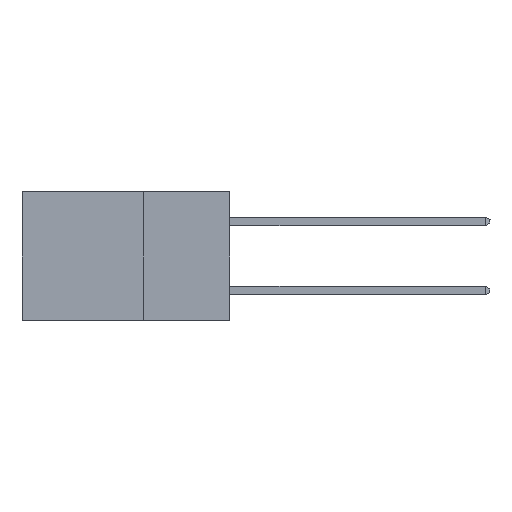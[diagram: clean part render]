
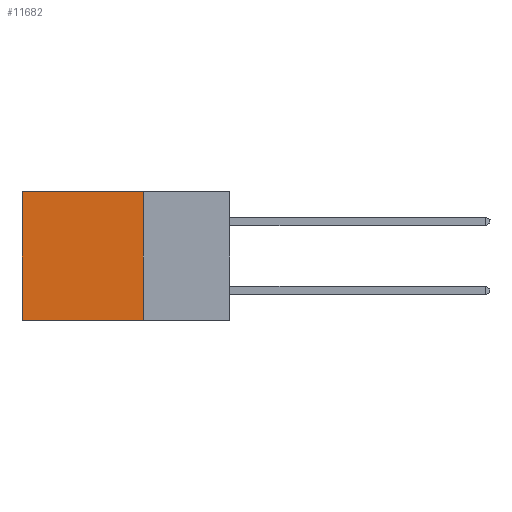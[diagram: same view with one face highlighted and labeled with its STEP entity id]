
A CAD part, left-side view. The second image highlights one B-rep face of the part: STEP entity #11682.
In plain terms, the highlighted planar face has unit normal (-1, 0, 0).
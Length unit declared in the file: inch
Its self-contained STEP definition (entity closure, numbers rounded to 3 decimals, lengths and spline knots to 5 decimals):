
#740 = VERTEX_POINT ( 'NONE', #20761 ) ;
#2469 = VECTOR ( 'NONE', #8230, 39.37008 ) ;
#3458 = ORIENTED_EDGE ( 'NONE', *, *, #10382, .F. ) ;
#4446 = EDGE_LOOP ( 'NONE', ( #15241, #3458, #6018, #7082 ) ) ;
#4618 = CARTESIAN_POINT ( 'NONE',  ( 0.2615, 0.25, -0.37 ) ) ;
#5547 = LINE ( 'NONE', #8915, #12121 ) ;
#6018 = ORIENTED_EDGE ( 'NONE', *, *, #13381, .F. ) ;
#6802 = VERTEX_POINT ( 'NONE', #23472 ) ;
#6805 = VECTOR ( 'NONE', #15416, 39.37008 ) ;
#6841 = FACE_OUTER_BOUND ( 'NONE', #4446, .T. ) ;
#7082 = ORIENTED_EDGE ( 'NONE', *, *, #19840, .T. ) ;
#7122 = DIRECTION ( 'NONE',  ( 0., 0., -1. ) ) ;
#7832 = VERTEX_POINT ( 'NONE', #16143 ) ;
#8230 = DIRECTION ( 'NONE',  ( 0., 1., 0. ) ) ;
#8915 = CARTESIAN_POINT ( 'NONE',  ( 0.2615, 0.25, -0.37 ) ) ;
#9118 = DIRECTION ( 'NONE',  ( 0., 0., -1. ) ) ;
#10382 = EDGE_CURVE ( 'NONE', #6802, #740, #13649, .T. ) ;
#11405 = CARTESIAN_POINT ( 'NONE',  ( 0.2615, 0.25, 0. ) ) ;
#11682 = ADVANCED_FACE ( 'NONE', ( #6841 ), #16119, .F. ) ;
#12121 = VECTOR ( 'NONE', #7122, 39.37008 ) ;
#12253 = VERTEX_POINT ( 'NONE', #11405 ) ;
#12734 = CARTESIAN_POINT ( 'NONE',  ( 0.2615, 0.25, -0.37 ) ) ;
#13381 = EDGE_CURVE ( 'NONE', #12253, #6802, #5547, .T. ) ;
#13649 = LINE ( 'NONE', #4618, #2469 ) ;
#14032 = AXIS2_PLACEMENT_3D ( 'NONE', #12734, #23703, #9118 ) ;
#14945 = VECTOR ( 'NONE', #15024, 39.37008 ) ;
#15024 = DIRECTION ( 'NONE',  ( 0., 1., 0. ) ) ;
#15241 = ORIENTED_EDGE ( 'NONE', *, *, #15618, .T. ) ;
#15416 = DIRECTION ( 'NONE',  ( 0., 0., -1. ) ) ;
#15618 = EDGE_CURVE ( 'NONE', #7832, #740, #20956, .T. ) ;
#16119 = PLANE ( 'NONE',  #14032 ) ;
#16143 = CARTESIAN_POINT ( 'NONE',  ( 0.2615, 0.6, 0. ) ) ;
#18393 = CARTESIAN_POINT ( 'NONE',  ( 0.2615, 0.25, 0. ) ) ;
#19014 = CARTESIAN_POINT ( 'NONE',  ( 0.2615, 0.6, -0.37 ) ) ;
#19840 = EDGE_CURVE ( 'NONE', #12253, #7832, #20689, .T. ) ;
#20689 = LINE ( 'NONE', #18393, #14945 ) ;
#20761 = CARTESIAN_POINT ( 'NONE',  ( 0.2615, 0.6, -0.37 ) ) ;
#20956 = LINE ( 'NONE', #19014, #6805 ) ;
#23472 = CARTESIAN_POINT ( 'NONE',  ( 0.2615, 0.25, -0.37 ) ) ;
#23703 = DIRECTION ( 'NONE',  ( 1., 0., 0. ) ) ;
